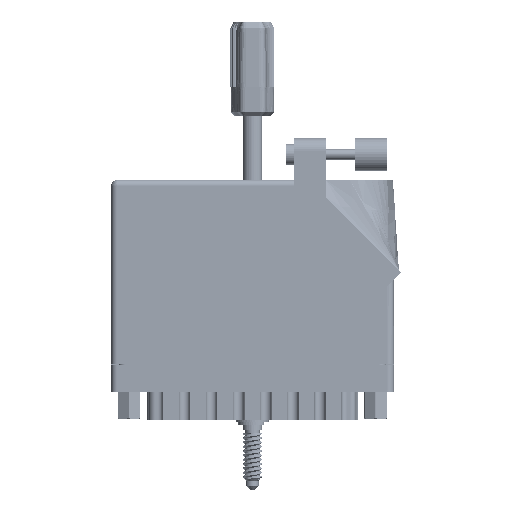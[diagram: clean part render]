
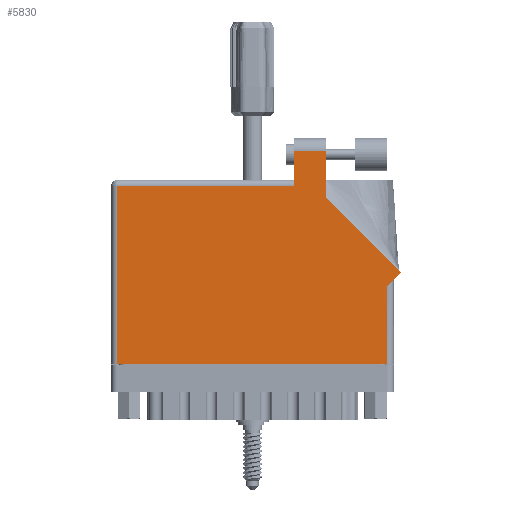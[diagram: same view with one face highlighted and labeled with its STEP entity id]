
A CAD part, front view. The second image highlights one B-rep face of the part: STEP entity #5830.
In plain terms, the highlighted face is planar.
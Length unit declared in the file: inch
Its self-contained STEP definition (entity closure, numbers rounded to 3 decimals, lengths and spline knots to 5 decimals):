
#1042 = CARTESIAN_POINT ( 'NONE',  ( 0.062, 1.713, 0. ) ) ;
#1467 = CARTESIAN_POINT ( 'NONE',  ( 2.656, 0.753, 0. ) ) ;
#4962 = VERTEX_POINT ( 'NONE', #92604 ) ;
#5143 = VECTOR ( 'NONE', #90306, 39.37008 ) ;
#5830 = ADVANCED_FACE ( 'NONE', ( #97885 ), #44761, .F. ) ;
#6652 = DIRECTION ( 'NONE',  ( -1., 0., 0. ) ) ;
#8380 = DIRECTION ( 'NONE',  ( 0., -1., 0. ) ) ;
#8386 = EDGE_CURVE ( 'NONE', #74207, #76537, #14299, .T. ) ;
#9235 = VERTEX_POINT ( 'NONE', #50711 ) ;
#14299 = LINE ( 'NONE', #83471, #80406 ) ;
#17983 = DIRECTION ( 'NONE',  ( 1., 0., 0. ) ) ;
#18563 = LINE ( 'NONE', #25129, #83155 ) ;
#19224 = ORIENTED_EDGE ( 'NONE', *, *, #61404, .T. ) ;
#22686 = CARTESIAN_POINT ( 'NONE',  ( 0., 1.775, 0. ) ) ;
#24031 = VERTEX_POINT ( 'NONE', #25867 ) ;
#25129 = CARTESIAN_POINT ( 'NONE',  ( 2.718, 0.815, 0. ) ) ;
#25865 = VECTOR ( 'NONE', #8380, 39.37008 ) ;
#25867 = CARTESIAN_POINT ( 'NONE',  ( 1.758, 1.713, 0. ) ) ;
#26709 = VERTEX_POINT ( 'NONE', #1467 ) ;
#28286 = EDGE_CURVE ( 'NONE', #24031, #73689, #97810, .T. ) ;
#28340 = AXIS2_PLACEMENT_3D ( 'NONE', #22686, #90373, #6652 ) ;
#32549 = CARTESIAN_POINT ( 'NONE',  ( 0., 0., 0. ) ) ;
#35699 = EDGE_CURVE ( 'NONE', #73689, #53899, #95459, .T. ) ;
#38861 = DIRECTION ( 'NONE',  ( 0., 1., 0. ) ) ;
#41326 = DIRECTION ( 'NONE',  ( -1., 0., 0. ) ) ;
#44761 = PLANE ( 'NONE',  #28340 ) ;
#47093 = LINE ( 'NONE', #32549, #81701 ) ;
#47654 = CARTESIAN_POINT ( 'NONE',  ( 2.78871, 0.88571, 0. ) ) ;
#50711 = CARTESIAN_POINT ( 'NONE',  ( 2.656, 0., 0. ) ) ;
#51724 = DIRECTION ( 'NONE',  ( -1., 0., 0. ) ) ;
#52725 = CARTESIAN_POINT ( 'NONE',  ( 2.656, 0.815, 0. ) ) ;
#53899 = VERTEX_POINT ( 'NONE', #75512 ) ;
#54252 = ORIENTED_EDGE ( 'NONE', *, *, #73901, .T. ) ;
#56187 = DIRECTION ( 'NONE',  ( -0.707, 0.707, 0. ) ) ;
#56273 = CARTESIAN_POINT ( 'NONE',  ( 2.065, 2.05, 0. ) ) ;
#57054 = CARTESIAN_POINT ( 'NONE',  ( 2.065, 1.60942, 0. ) ) ;
#61404 = EDGE_CURVE ( 'NONE', #26709, #96996, #18563, .T. ) ;
#61644 = ORIENTED_EDGE ( 'NONE', *, *, #83005, .T. ) ;
#62429 = CARTESIAN_POINT ( 'NONE',  ( 1.758, 2.05, 0. ) ) ;
#64948 = VECTOR ( 'NONE', #65402, 39.37008 ) ;
#65064 = EDGE_CURVE ( 'NONE', #4962, #24031, #92605, .T. ) ;
#65402 = DIRECTION ( 'NONE',  ( 0., -1., 0. ) ) ;
#68068 = CARTESIAN_POINT ( 'NONE',  ( 1.758, 1.775, 0. ) ) ;
#68975 = ORIENTED_EDGE ( 'NONE', *, *, #28286, .T. ) ;
#69177 = EDGE_CURVE ( 'NONE', #53899, #9235, #47093, .T. ) ;
#71343 = ORIENTED_EDGE ( 'NONE', *, *, #88919, .T. ) ;
#73689 = VERTEX_POINT ( 'NONE', #1042 ) ;
#73901 = EDGE_CURVE ( 'NONE', #96996, #74207, #86718, .T. ) ;
#74207 = VERTEX_POINT ( 'NONE', #57054 ) ;
#74537 = VECTOR ( 'NONE', #41326, 39.37008 ) ;
#75512 = CARTESIAN_POINT ( 'NONE',  ( 0.062, 0., 0. ) ) ;
#75518 = ORIENTED_EDGE ( 'NONE', *, *, #65064, .T. ) ;
#76537 = VERTEX_POINT ( 'NONE', #56273 ) ;
#76886 = VECTOR ( 'NONE', #51724, 39.37008 ) ;
#77432 = EDGE_LOOP ( 'NONE', ( #86044, #71343, #75518, #68975, #95019, #89928, #61644, #19224, #54252 ) ) ;
#78905 = LINE ( 'NONE', #62429, #74537 ) ;
#79210 = DIRECTION ( 'NONE',  ( 0.707, 0.707, 0. ) ) ;
#80406 = VECTOR ( 'NONE', #38861, 39.37008 ) ;
#81701 = VECTOR ( 'NONE', #17983, 39.37008 ) ;
#82277 = CARTESIAN_POINT ( 'NONE',  ( 0., 1.713, 0. ) ) ;
#83005 = EDGE_CURVE ( 'NONE', #9235, #26709, #97821, .T. ) ;
#83155 = VECTOR ( 'NONE', #79210, 39.37008 ) ;
#83471 = CARTESIAN_POINT ( 'NONE',  ( 2.065, 1.60942, 0. ) ) ;
#83721 = VECTOR ( 'NONE', #56187, 39.37008 ) ;
#86044 = ORIENTED_EDGE ( 'NONE', *, *, #8386, .T. ) ;
#86718 = LINE ( 'NONE', #47654, #83721 ) ;
#87441 = CARTESIAN_POINT ( 'NONE',  ( 0.062, 0., 0. ) ) ;
#88919 = EDGE_CURVE ( 'NONE', #76537, #4962, #78905, .T. ) ;
#89928 = ORIENTED_EDGE ( 'NONE', *, *, #69177, .T. ) ;
#90306 = DIRECTION ( 'NONE',  ( 0., 1., 0. ) ) ;
#90373 = DIRECTION ( 'NONE',  ( 0., 0., -1. ) ) ;
#92604 = CARTESIAN_POINT ( 'NONE',  ( 1.758, 2.05, 0. ) ) ;
#92605 = LINE ( 'NONE', #68068, #25865 ) ;
#94047 = CARTESIAN_POINT ( 'NONE',  ( 2.78871, 0.88571, 0. ) ) ;
#95019 = ORIENTED_EDGE ( 'NONE', *, *, #35699, .T. ) ;
#95459 = LINE ( 'NONE', #87441, #64948 ) ;
#96996 = VERTEX_POINT ( 'NONE', #94047 ) ;
#97810 = LINE ( 'NONE', #82277, #76886 ) ;
#97821 = LINE ( 'NONE', #52725, #5143 ) ;
#97885 = FACE_OUTER_BOUND ( 'NONE', #77432, .T. ) ;
